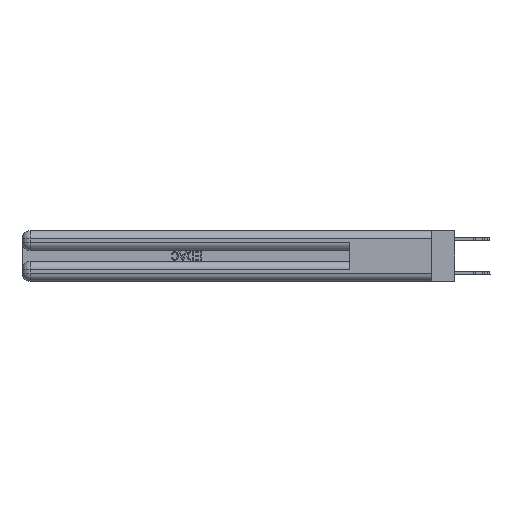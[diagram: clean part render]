
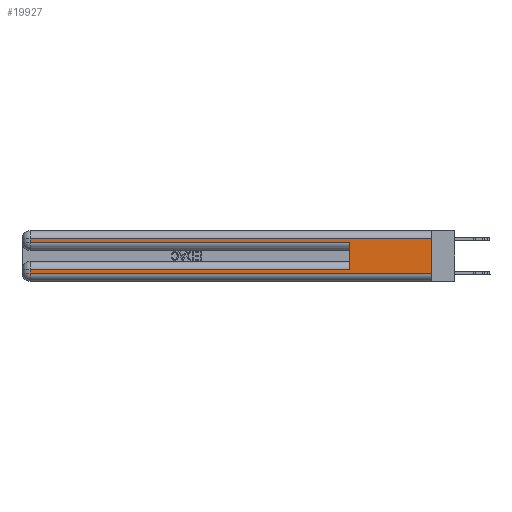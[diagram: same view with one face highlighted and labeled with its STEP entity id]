
A CAD part, left-side view. The second image highlights one B-rep face of the part: STEP entity #19927.
In plain terms, the highlighted planar face has unit normal (-1, 0, 0).
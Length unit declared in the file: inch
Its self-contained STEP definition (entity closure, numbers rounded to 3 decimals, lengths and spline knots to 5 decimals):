
#400 = VECTOR ( 'NONE', #35068, 39.37008 ) ;
#1134 = LINE ( 'NONE', #32450, #3177 ) ;
#1517 = DIRECTION ( 'NONE',  ( 0., -1., 0. ) ) ;
#1866 = DIRECTION ( 'NONE',  ( 0., 0., -1. ) ) ;
#2751 = PLANE ( 'NONE',  #4918 ) ;
#3177 = VECTOR ( 'NONE', #15282, 39.37008 ) ;
#4913 = CARTESIAN_POINT ( 'NONE',  ( 0., 0., 0.06 ) ) ;
#4918 = AXIS2_PLACEMENT_3D ( 'NONE', #14263, #25764, #26322 ) ;
#5437 = CARTESIAN_POINT ( 'NONE',  ( 0., 2.94, 0.37 ) ) ;
#7533 = CARTESIAN_POINT ( 'NONE',  ( 0., 2.94, 0.37 ) ) ;
#7592 = VERTEX_POINT ( 'NONE', #19485 ) ;
#8298 = ORIENTED_EDGE ( 'NONE', *, *, #14619, .F. ) ;
#8650 = DIRECTION ( 'NONE',  ( 0., 0., -1. ) ) ;
#8727 = EDGE_CURVE ( 'NONE', #31819, #19848, #10185, .T. ) ;
#8741 = LINE ( 'NONE', #17595, #28186 ) ;
#8868 = VERTEX_POINT ( 'NONE', #28083 ) ;
#9391 = LINE ( 'NONE', #20886, #33831 ) ;
#9556 = VERTEX_POINT ( 'NONE', #14186 ) ;
#10185 = LINE ( 'NONE', #7533, #33097 ) ;
#11070 = CARTESIAN_POINT ( 'NONE',  ( 0., 0., 0.31 ) ) ;
#12945 = EDGE_LOOP ( 'NONE', ( #8298, #27924, #35424, #18055, #26791, #19580, #28885, #24343 ) ) ;
#13722 = EDGE_CURVE ( 'NONE', #33760, #7592, #8741, .T. ) ;
#14186 = CARTESIAN_POINT ( 'NONE',  ( 0., 0.6, 0.285 ) ) ;
#14263 = CARTESIAN_POINT ( 'NONE',  ( 0., 0., 0.37 ) ) ;
#14311 = LINE ( 'NONE', #5437, #27651 ) ;
#14535 = LINE ( 'NONE', #26410, #400 ) ;
#14619 = EDGE_CURVE ( 'NONE', #33760, #28214, #25063, .T. ) ;
#14673 = EDGE_CURVE ( 'NONE', #7592, #8868, #14311, .T. ) ;
#15282 = DIRECTION ( 'NONE',  ( 0., 0., 1. ) ) ;
#15613 = VECTOR ( 'NONE', #1517, 39.37008 ) ;
#16195 = CARTESIAN_POINT ( 'NONE',  ( 0., 0., 0.37 ) ) ;
#17595 = CARTESIAN_POINT ( 'NONE',  ( 0., 0., 0.31 ) ) ;
#18055 = ORIENTED_EDGE ( 'NONE', *, *, #33612, .T. ) ;
#19485 = CARTESIAN_POINT ( 'NONE',  ( 0., 2.94, 0.31 ) ) ;
#19580 = ORIENTED_EDGE ( 'NONE', *, *, #25682, .T. ) ;
#19848 = VERTEX_POINT ( 'NONE', #22741 ) ;
#19927 = ADVANCED_FACE ( 'NONE', ( #28591 ), #2751, .F. ) ;
#20153 = DIRECTION ( 'NONE',  ( 0., -1., 0. ) ) ;
#20240 = DIRECTION ( 'NONE',  ( 0., 1., 0. ) ) ;
#20886 = CARTESIAN_POINT ( 'NONE',  ( 0., 0., 0.285 ) ) ;
#22741 = CARTESIAN_POINT ( 'NONE',  ( 0., 2.94, 0.06 ) ) ;
#23078 = CARTESIAN_POINT ( 'NONE',  ( 0., 0., 0.06 ) ) ;
#23903 = CARTESIAN_POINT ( 'NONE',  ( 0., 0.6, 0.085 ) ) ;
#24343 = ORIENTED_EDGE ( 'NONE', *, *, #30672, .T. ) ;
#25063 = LINE ( 'NONE', #16195, #31850 ) ;
#25282 = LINE ( 'NONE', #4913, #15613 ) ;
#25682 = EDGE_CURVE ( 'NONE', #33718, #31819, #14535, .T. ) ;
#25764 = DIRECTION ( 'NONE',  ( 1., 0., 0. ) ) ;
#26322 = DIRECTION ( 'NONE',  ( 0., 0., -1. ) ) ;
#26410 = CARTESIAN_POINT ( 'NONE',  ( 0., 0., 0.085 ) ) ;
#26791 = ORIENTED_EDGE ( 'NONE', *, *, #36368, .F. ) ;
#27651 = VECTOR ( 'NONE', #8650, 39.37008 ) ;
#27924 = ORIENTED_EDGE ( 'NONE', *, *, #13722, .T. ) ;
#28083 = CARTESIAN_POINT ( 'NONE',  ( 0., 2.94, 0.285 ) ) ;
#28186 = VECTOR ( 'NONE', #20240, 39.37008 ) ;
#28214 = VERTEX_POINT ( 'NONE', #23078 ) ;
#28591 = FACE_OUTER_BOUND ( 'NONE', #12945, .T. ) ;
#28885 = ORIENTED_EDGE ( 'NONE', *, *, #8727, .T. ) ;
#30672 = EDGE_CURVE ( 'NONE', #19848, #28214, #25282, .T. ) ;
#31819 = VERTEX_POINT ( 'NONE', #32290 ) ;
#31850 = VECTOR ( 'NONE', #1866, 39.37008 ) ;
#32290 = CARTESIAN_POINT ( 'NONE',  ( 0., 2.94, 0.085 ) ) ;
#32450 = CARTESIAN_POINT ( 'NONE',  ( 0., 0.6, 0.145 ) ) ;
#33097 = VECTOR ( 'NONE', #36382, 39.37008 ) ;
#33612 = EDGE_CURVE ( 'NONE', #8868, #9556, #9391, .T. ) ;
#33718 = VERTEX_POINT ( 'NONE', #23903 ) ;
#33760 = VERTEX_POINT ( 'NONE', #11070 ) ;
#33831 = VECTOR ( 'NONE', #20153, 39.37008 ) ;
#35068 = DIRECTION ( 'NONE',  ( 0., 1., 0. ) ) ;
#35424 = ORIENTED_EDGE ( 'NONE', *, *, #14673, .T. ) ;
#36368 = EDGE_CURVE ( 'NONE', #33718, #9556, #1134, .T. ) ;
#36382 = DIRECTION ( 'NONE',  ( 0., 0., -1. ) ) ;
